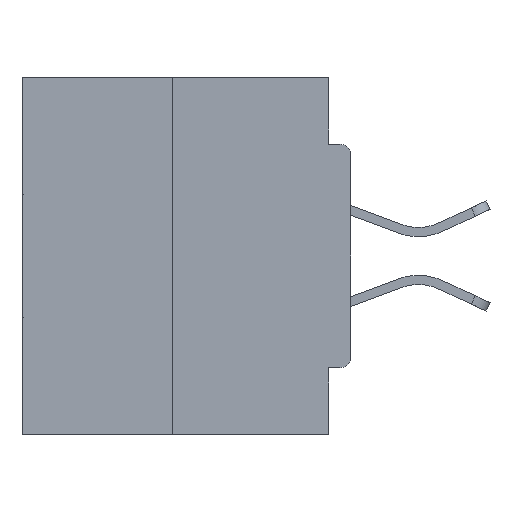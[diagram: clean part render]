
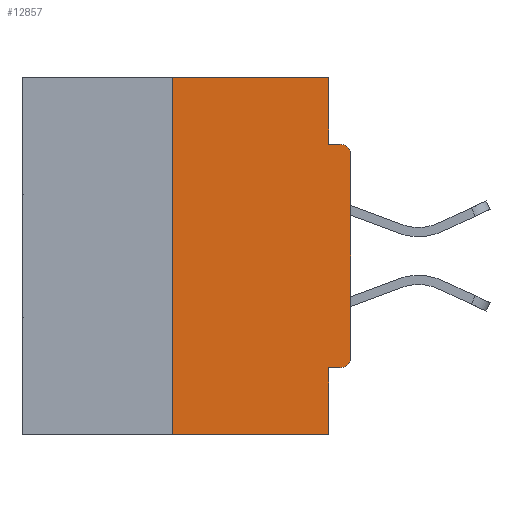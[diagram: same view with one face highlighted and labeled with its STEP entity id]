
A CAD part, left-side view. The second image highlights one B-rep face of the part: STEP entity #12857.
In plain terms, the highlighted planar face has unit normal (-1, 0, 0).
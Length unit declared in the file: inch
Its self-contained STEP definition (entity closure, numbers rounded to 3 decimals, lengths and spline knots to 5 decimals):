
#177 = VERTEX_POINT ( 'NONE', #37933 ) ;
#417 = LINE ( 'NONE', #32723, #5509 ) ;
#809 = CARTESIAN_POINT ( 'NONE',  ( 0., 0.031, -0.4065 ) ) ;
#813 = EDGE_CURVE ( 'NONE', #21555, #3152, #11325, .T. ) ;
#1594 = CARTESIAN_POINT ( 'NONE',  ( 0., 0.46, -0.5 ) ) ;
#3152 = VERTEX_POINT ( 'NONE', #17802 ) ;
#4379 = CARTESIAN_POINT ( 'NONE',  ( 0., 0.25, 0. ) ) ;
#4767 = AXIS2_PLACEMENT_3D ( 'NONE', #5618, #35356, #8696 ) ;
#5509 = VECTOR ( 'NONE', #27272, 39.37008 ) ;
#5618 = CARTESIAN_POINT ( 'NONE',  ( 0., 0.015, -0.1085 ) ) ;
#5912 = DIRECTION ( 'NONE',  ( 0., -1., 0. ) ) ;
#6774 = DIRECTION ( 'NONE',  ( 0., 0., -1. ) ) ;
#6882 = CARTESIAN_POINT ( 'NONE',  ( 0., 0.031, -0.0935 ) ) ;
#7254 = ORIENTED_EDGE ( 'NONE', *, *, #15822, .T. ) ;
#8092 = ORIENTED_EDGE ( 'NONE', *, *, #12834, .F. ) ;
#8208 = LINE ( 'NONE', #8942, #19250 ) ;
#8283 = EDGE_CURVE ( 'NONE', #29445, #177, #8208, .T. ) ;
#8696 = DIRECTION ( 'NONE',  ( 0., 0., -1. ) ) ;
#8933 = ORIENTED_EDGE ( 'NONE', *, *, #34945, .T. ) ;
#8942 = CARTESIAN_POINT ( 'NONE',  ( 0., 0., -0.0935 ) ) ;
#10982 = EDGE_CURVE ( 'NONE', #33965, #32790, #17490, .T. ) ;
#11110 = VECTOR ( 'NONE', #5912, 39.37008 ) ;
#11325 = LINE ( 'NONE', #23219, #11110 ) ;
#11362 = LINE ( 'NONE', #14128, #28899 ) ;
#11737 = VECTOR ( 'NONE', #6774, 39.37008 ) ;
#12178 = CARTESIAN_POINT ( 'NONE',  ( 0., 0.25, -0.5 ) ) ;
#12289 = EDGE_CURVE ( 'NONE', #15148, #24636, #27616, .T. ) ;
#12442 = CARTESIAN_POINT ( 'NONE',  ( 0., 0., -0.3915 ) ) ;
#12834 = EDGE_CURVE ( 'NONE', #26694, #21555, #11362, .T. ) ;
#12857 = ADVANCED_FACE ( 'NONE', ( #25829 ), #13545, .F. ) ;
#13440 = CIRCLE ( 'NONE', #4767, 0.015 ) ;
#13545 = PLANE ( 'NONE',  #32623 ) ;
#14128 = CARTESIAN_POINT ( 'NONE',  ( 0., 0.25, 0. ) ) ;
#14868 = ORIENTED_EDGE ( 'NONE', *, *, #24569, .F. ) ;
#15148 = VERTEX_POINT ( 'NONE', #12442 ) ;
#15822 = EDGE_CURVE ( 'NONE', #24636, #177, #13440, .T. ) ;
#16701 = EDGE_LOOP ( 'NONE', ( #24319, #8092, #21531, #20392, #14868, #8933, #33860, #7254, #18971, #36262 ) ) ;
#17490 = LINE ( 'NONE', #38144, #11737 ) ;
#17802 = CARTESIAN_POINT ( 'NONE',  ( 0., 0.031, 0. ) ) ;
#18971 = ORIENTED_EDGE ( 'NONE', *, *, #8283, .F. ) ;
#19250 = VECTOR ( 'NONE', #32508, 39.37008 ) ;
#19400 = DIRECTION ( 'NONE',  ( 0., 1., 0. ) ) ;
#19516 = VECTOR ( 'NONE', #22184, 39.37008 ) ;
#20392 = ORIENTED_EDGE ( 'NONE', *, *, #10982, .F. ) ;
#21531 = ORIENTED_EDGE ( 'NONE', *, *, #35323, .T. ) ;
#21539 = CARTESIAN_POINT ( 'NONE',  ( 0., 0.015, -0.4065 ) ) ;
#21555 = VERTEX_POINT ( 'NONE', #4379 ) ;
#22184 = DIRECTION ( 'NONE',  ( 0., 0., 1. ) ) ;
#22991 = CIRCLE ( 'NONE', #33544, 0.015 ) ;
#23081 = CARTESIAN_POINT ( 'NONE',  ( 0., 0.46, 0. ) ) ;
#23219 = CARTESIAN_POINT ( 'NONE',  ( 0., 0.46, 0. ) ) ;
#23260 = DIRECTION ( 'NONE',  ( 0., 0., 1. ) ) ;
#24319 = ORIENTED_EDGE ( 'NONE', *, *, #813, .F. ) ;
#24569 = EDGE_CURVE ( 'NONE', #36259, #33965, #34559, .T. ) ;
#24636 = VERTEX_POINT ( 'NONE', #37479 ) ;
#25629 = CARTESIAN_POINT ( 'NONE',  ( 0., 0., -0.4065 ) ) ;
#25829 = FACE_OUTER_BOUND ( 'NONE', #16701, .T. ) ;
#25856 = VECTOR ( 'NONE', #19400, 39.37008 ) ;
#26694 = VERTEX_POINT ( 'NONE', #12178 ) ;
#27272 = DIRECTION ( 'NONE',  ( 0., 0., -1. ) ) ;
#27557 = DIRECTION ( 'NONE',  ( 0., 0., -1. ) ) ;
#27616 = LINE ( 'NONE', #33469, #19516 ) ;
#27868 = DIRECTION ( 'NONE',  ( 0., -1., 0. ) ) ;
#28599 = EDGE_CURVE ( 'NONE', #3152, #29445, #417, .T. ) ;
#28899 = VECTOR ( 'NONE', #23260, 39.37008 ) ;
#29282 = CARTESIAN_POINT ( 'NONE',  ( 0., 0.031, -0.5 ) ) ;
#29445 = VERTEX_POINT ( 'NONE', #6882 ) ;
#30888 = CARTESIAN_POINT ( 'NONE',  ( 0., 0.015, -0.3915 ) ) ;
#31729 = VECTOR ( 'NONE', #27868, 39.37008 ) ;
#31860 = DIRECTION ( 'NONE',  ( 0., 0., -1. ) ) ;
#32508 = DIRECTION ( 'NONE',  ( 0., -1., 0. ) ) ;
#32623 = AXIS2_PLACEMENT_3D ( 'NONE', #23081, #37312, #31860 ) ;
#32723 = CARTESIAN_POINT ( 'NONE',  ( 0., 0.031, 0. ) ) ;
#32790 = VERTEX_POINT ( 'NONE', #29282 ) ;
#33469 = CARTESIAN_POINT ( 'NONE',  ( 0., 0., 0. ) ) ;
#33544 = AXIS2_PLACEMENT_3D ( 'NONE', #30888, #33982, #27557 ) ;
#33860 = ORIENTED_EDGE ( 'NONE', *, *, #12289, .T. ) ;
#33965 = VERTEX_POINT ( 'NONE', #809 ) ;
#33982 = DIRECTION ( 'NONE',  ( -1., 0., 0. ) ) ;
#34083 = LINE ( 'NONE', #1594, #31729 ) ;
#34559 = LINE ( 'NONE', #25629, #25856 ) ;
#34945 = EDGE_CURVE ( 'NONE', #36259, #15148, #22991, .T. ) ;
#35323 = EDGE_CURVE ( 'NONE', #26694, #32790, #34083, .T. ) ;
#35356 = DIRECTION ( 'NONE',  ( -1., 0., 0. ) ) ;
#36259 = VERTEX_POINT ( 'NONE', #21539 ) ;
#36262 = ORIENTED_EDGE ( 'NONE', *, *, #28599, .F. ) ;
#37312 = DIRECTION ( 'NONE',  ( 1., 0., 0. ) ) ;
#37479 = CARTESIAN_POINT ( 'NONE',  ( 0., 0., -0.1085 ) ) ;
#37933 = CARTESIAN_POINT ( 'NONE',  ( 0., 0.015, -0.0935 ) ) ;
#38144 = CARTESIAN_POINT ( 'NONE',  ( 0., 0.031, -0.5 ) ) ;
